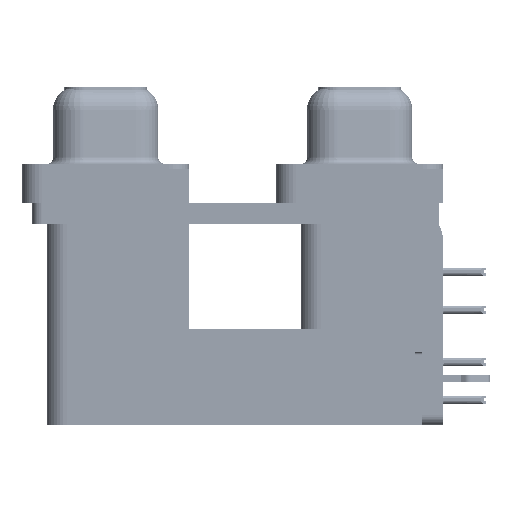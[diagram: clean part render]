
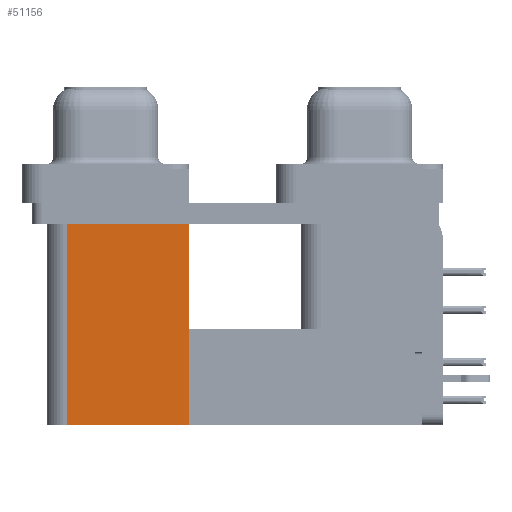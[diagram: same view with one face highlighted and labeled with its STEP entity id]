
A CAD part, left-side view. The second image highlights one B-rep face of the part: STEP entity #51156.
In plain terms, the highlighted planar face has unit normal (-1, 0, 0).
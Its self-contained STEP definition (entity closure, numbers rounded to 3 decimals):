
#662 = CARTESIAN_POINT ( 'NONE',  ( 3.7, 12.775, -19.2 ) ) ;
#2072 = LINE ( 'NONE', #22209, #12954 ) ;
#3584 = VECTOR ( 'NONE', #41713, 1000. ) ;
#8069 = CARTESIAN_POINT ( 'NONE',  ( 3.7, 21.975, -19.2 ) ) ;
#8631 = DIRECTION ( 'NONE',  ( 0., 1., 0. ) ) ;
#12547 = ORIENTED_EDGE ( 'NONE', *, *, #18070, .F. ) ;
#12954 = VECTOR ( 'NONE', #21293, 1000. ) ;
#13233 = ORIENTED_EDGE ( 'NONE', *, *, #29621, .T. ) ;
#15271 = AXIS2_PLACEMENT_3D ( 'NONE', #18083, #60675, #8631 ) ;
#18070 = EDGE_CURVE ( 'NONE', #41332, #32781, #21558, .T. ) ;
#18083 = CARTESIAN_POINT ( 'NONE',  ( 3.7, 12.775, -19.2 ) ) ;
#21293 = DIRECTION ( 'NONE',  ( 0., 1., 0. ) ) ;
#21558 = LINE ( 'NONE', #50553, #3584 ) ;
#22209 = CARTESIAN_POINT ( 'NONE',  ( 3.7, 12.775, -2.5 ) ) ;
#22250 = EDGE_CURVE ( 'NONE', #56602, #30136, #2072, .T. ) ;
#22505 = VECTOR ( 'NONE', #60004, 1000. ) ;
#26442 = LINE ( 'NONE', #52609, #32474 ) ;
#26609 = PLANE ( 'NONE',  #15271 ) ;
#26918 = FACE_OUTER_BOUND ( 'NONE', #36594, .T. ) ;
#27143 = CARTESIAN_POINT ( 'NONE',  ( 3.7, 21.975, -2.5 ) ) ;
#29621 = EDGE_CURVE ( 'NONE', #41332, #56602, #26442, .T. ) ;
#30136 = VERTEX_POINT ( 'NONE', #27143 ) ;
#32474 = VECTOR ( 'NONE', #47222, 1000. ) ;
#32781 = VERTEX_POINT ( 'NONE', #8069 ) ;
#36594 = EDGE_LOOP ( 'NONE', ( #42660, #59564, #12547, #13233 ) ) ;
#36633 = CARTESIAN_POINT ( 'NONE',  ( 3.7, 21.975, -19.2 ) ) ;
#37475 = CARTESIAN_POINT ( 'NONE',  ( 3.7, 12.775, -2.5 ) ) ;
#41332 = VERTEX_POINT ( 'NONE', #662 ) ;
#41713 = DIRECTION ( 'NONE',  ( 0., 1., 0. ) ) ;
#42660 = ORIENTED_EDGE ( 'NONE', *, *, #22250, .T. ) ;
#47222 = DIRECTION ( 'NONE',  ( 0., 0., 1. ) ) ;
#47475 = EDGE_CURVE ( 'NONE', #32781, #30136, #48666, .T. ) ;
#48666 = LINE ( 'NONE', #36633, #22505 ) ;
#50553 = CARTESIAN_POINT ( 'NONE',  ( 3.7, 12.775, -19.2 ) ) ;
#51156 = ADVANCED_FACE ( 'NONE', ( #26918 ), #26609, .F. ) ;
#52609 = CARTESIAN_POINT ( 'NONE',  ( 3.7, 12.775, -19.2 ) ) ;
#56602 = VERTEX_POINT ( 'NONE', #37475 ) ;
#59564 = ORIENTED_EDGE ( 'NONE', *, *, #47475, .F. ) ;
#60004 = DIRECTION ( 'NONE',  ( 0., 0., 1. ) ) ;
#60675 = DIRECTION ( 'NONE',  ( 1., 0., 0. ) ) ;
